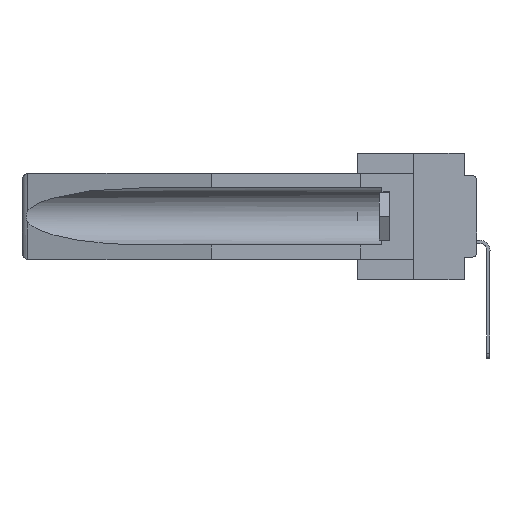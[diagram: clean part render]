
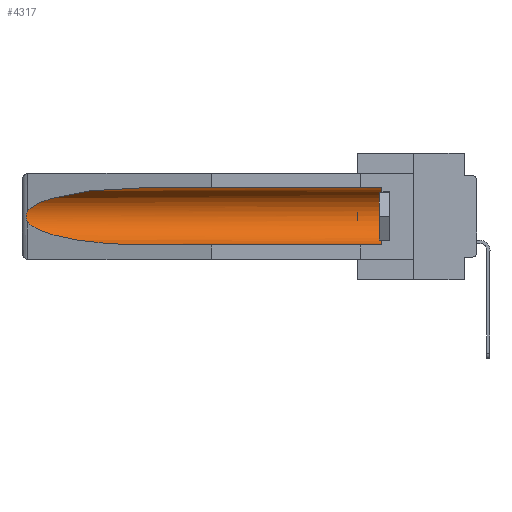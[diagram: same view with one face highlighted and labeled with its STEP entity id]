
A CAD part, left-side view. The second image highlights one B-rep face of the part: STEP entity #4317.
In plain terms, the highlighted cylindrical face has radius 2.857 mm (diameter 5.715 mm), a partial arc.
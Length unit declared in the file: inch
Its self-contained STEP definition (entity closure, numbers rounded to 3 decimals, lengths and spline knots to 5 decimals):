
#80 = ORIENTED_EDGE ( 'NONE', *, *, #23059, .T. ) ;
#447 = VERTEX_POINT ( 'NONE', #25496 ) ;
#1907 = FACE_OUTER_BOUND ( 'NONE', #30449, .T. ) ;
#1928 = CARTESIAN_POINT ( 'NONE',  ( 0.26655, 1.53094, -0.18657 ) ) ;
#2059 = CARTESIAN_POINT ( 'NONE',  ( 0.2673, 1.53269, -0.17917 ) ) ;
#2825 = CARTESIAN_POINT ( 'NONE',  ( 0.155, -0.30754, -0.284 ) ) ;
#3562 = CARTESIAN_POINT ( 'NONE',  ( 0.155, 0.126, -0.059 ) ) ;
#4317 = ADVANCED_FACE ( 'NONE', ( #1907 ), #10285, .F. ) ;
#4556 = CARTESIAN_POINT ( 'NONE',  ( 0.26537, 1.52718, -0.19328 ) ) ;
#4923 = CARTESIAN_POINT ( 'NONE',  ( 0.26537, 1.52718, -0.14972 ) ) ;
#10285 = CYLINDRICAL_SURFACE ( 'NONE', #39070, 0.1125 ) ;
#11427 = CARTESIAN_POINT ( 'NONE',  ( 0.26597, 1.5296, -0.19026 ) ) ;
#12116 = DIRECTION ( 'NONE',  ( 0., 1., 0. ) ) ;
#12174 = CARTESIAN_POINT ( 'NONE',  ( 0.21114, 1.30732, -0.284 ) ) ;
#13709 = CARTESIAN_POINT ( 'NONE',  ( 0.155, 1.07973, -0.059 ) ) ;
#14213 = CARTESIAN_POINT ( 'NONE',  ( 0.26537, 1.52718, -0.14972 ) ) ;
#14276 =( BOUNDED_CURVE ( )  B_SPLINE_CURVE ( 3, ( #17224, #33228, #26645, #4923 ),
 .UNSPECIFIED., .F., .F. ) 
 B_SPLINE_CURVE_WITH_KNOTS ( ( 4, 4 ),
 ( 4.71239, 6.08839 ),
 .UNSPECIFIED. ) 
 CURVE ( )  GEOMETRIC_REPRESENTATION_ITEM ( )  RATIONAL_B_SPLINE_CURVE ( ( 1., 0.848, 0.848, 1. ) ) 
 REPRESENTATION_ITEM ( '' )  );
#14477 = CARTESIAN_POINT ( 'NONE',  ( 0.2673, 1.5327, -0.16383 ) ) ;
#14496 =( BOUNDED_CURVE ( )  B_SPLINE_CURVE ( 3, ( #40096, #40370, #12174, #34138 ),
 .UNSPECIFIED., .F., .F. ) 
 B_SPLINE_CURVE_WITH_KNOTS ( ( 4, 4 ),
 ( 0.1948, 1.5708 ),
 .UNSPECIFIED. ) 
 CURVE ( )  GEOMETRIC_REPRESENTATION_ITEM ( )  RATIONAL_B_SPLINE_CURVE ( ( 1., 0.848, 0.848, 1. ) ) 
 REPRESENTATION_ITEM ( '' )  );
#15516 = EDGE_CURVE ( 'NONE', #447, #30851, #26678, .T. ) ;
#17025 = EDGE_CURVE ( 'NONE', #30851, #34064, #31449, .T. ) ;
#17224 = CARTESIAN_POINT ( 'NONE',  ( 0.155, 1.07973, -0.059 ) ) ;
#17232 = VECTOR ( 'NONE', #18819, 39.37008 ) ;
#17398 = CARTESIAN_POINT ( 'NONE',  ( 0.2675, 1.53308, -0.16763 ) ) ;
#18125 = CARTESIAN_POINT ( 'NONE',  ( 0.155, 1.07973, -0.284 ) ) ;
#18819 = DIRECTION ( 'NONE',  ( 0., 1., 0. ) ) ;
#19280 = DIRECTION ( 'NONE',  ( 0., 0., 1. ) ) ;
#20169 = VECTOR ( 'NONE', #32466, 39.37008 ) ;
#20785 = CARTESIAN_POINT ( 'NONE',  ( 0.2675, 1.53308, -0.17534 ) ) ;
#21866 = ORIENTED_EDGE ( 'NONE', *, *, #29624, .F. ) ;
#22218 = EDGE_CURVE ( 'NONE', #34064, #33865, #14276, .T. ) ;
#22240 = ORIENTED_EDGE ( 'NONE', *, *, #17025, .T. ) ;
#23059 = EDGE_CURVE ( 'NONE', #33107, #29439, #14496, .T. ) ;
#24380 = DIRECTION ( 'NONE',  ( 0., 0., 1. ) ) ;
#25030 = CARTESIAN_POINT ( 'NONE',  ( 0.26537, 1.52718, -0.14972 ) ) ;
#25496 = CARTESIAN_POINT ( 'NONE',  ( 0.155, 0.126, -0.284 ) ) ;
#26645 = CARTESIAN_POINT ( 'NONE',  ( 0.25451, 1.48313, -0.09465 ) ) ;
#26678 = CIRCLE ( 'NONE', #33029, 0.1125 ) ;
#27065 = CARTESIAN_POINT ( 'NONE',  ( 0.26597, 1.52961, -0.15275 ) ) ;
#29420 = CARTESIAN_POINT ( 'NONE',  ( 0.155, -0.30754, -0.059 ) ) ;
#29439 = VERTEX_POINT ( 'NONE', #18125 ) ;
#29624 = EDGE_CURVE ( 'NONE', #447, #29439, #34885, .T. ) ;
#30449 = EDGE_LOOP ( 'NONE', ( #37725, #36989, #80, #21866, #32285, #22240 ) ) ;
#30478 = EDGE_CURVE ( 'NONE', #33865, #33107, #39978, .T. ) ;
#30646 = CARTESIAN_POINT ( 'NONE',  ( 0.155, 0.126, -0.1715 ) ) ;
#30851 = VERTEX_POINT ( 'NONE', #3562 ) ;
#30903 = CARTESIAN_POINT ( 'NONE',  ( 0.155, -0.30754, -0.1715 ) ) ;
#30908 = CARTESIAN_POINT ( 'NONE',  ( 0.26537, 1.52718, -0.19328 ) ) ;
#31449 = LINE ( 'NONE', #29420, #20169 ) ;
#32285 = ORIENTED_EDGE ( 'NONE', *, *, #15516, .T. ) ;
#32466 = DIRECTION ( 'NONE',  ( 0., 1., 0. ) ) ;
#33029 = AXIS2_PLACEMENT_3D ( 'NONE', #30646, #40732, #24380 ) ;
#33107 = VERTEX_POINT ( 'NONE', #30908 ) ;
#33228 = CARTESIAN_POINT ( 'NONE',  ( 0.21114, 1.30732, -0.059 ) ) ;
#33865 = VERTEX_POINT ( 'NONE', #25030 ) ;
#34064 = VERTEX_POINT ( 'NONE', #13709 ) ;
#34138 = CARTESIAN_POINT ( 'NONE',  ( 0.155, 1.07973, -0.284 ) ) ;
#34885 = LINE ( 'NONE', #2825, #17232 ) ;
#36304 = CARTESIAN_POINT ( 'NONE',  ( 0.26654, 1.53092, -0.15636 ) ) ;
#36989 = ORIENTED_EDGE ( 'NONE', *, *, #30478, .T. ) ;
#37725 = ORIENTED_EDGE ( 'NONE', *, *, #22218, .T. ) ;
#39070 = AXIS2_PLACEMENT_3D ( 'NONE', #30903, #12116, #19280 ) ;
#39978 = B_SPLINE_CURVE_WITH_KNOTS ( 'NONE', 3,
 ( #14213, #27065, #36304, #14477, #17398, #20785, #2059, #1928, #11427, #4556 ),
 .UNSPECIFIED., .F., .F.,
 ( 4, 2, 2, 2, 4 ),
 ( 0., 0.00029, 0.00058, 0.00087, 0.00117 ),
 .UNSPECIFIED. ) ;
#40096 = CARTESIAN_POINT ( 'NONE',  ( 0.26537, 1.52718, -0.19328 ) ) ;
#40370 = CARTESIAN_POINT ( 'NONE',  ( 0.25451, 1.48313, -0.24835 ) ) ;
#40732 = DIRECTION ( 'NONE',  ( 0., -1., 0. ) ) ;
